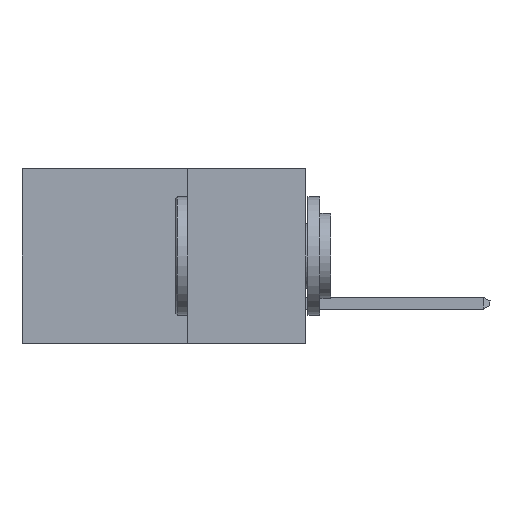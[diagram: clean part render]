
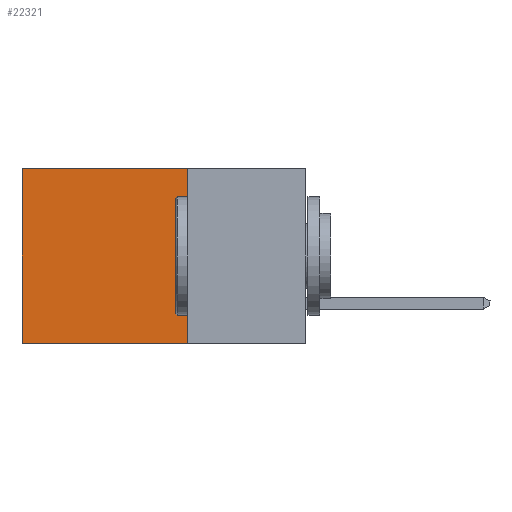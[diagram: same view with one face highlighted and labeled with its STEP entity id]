
A CAD part, left-side view. The second image highlights one B-rep face of the part: STEP entity #22321.
In plain terms, the highlighted planar face has unit normal (-1, 0, 0).
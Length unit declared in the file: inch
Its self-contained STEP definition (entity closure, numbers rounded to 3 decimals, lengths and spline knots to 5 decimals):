
#31 = AXIS2_PLACEMENT_3D ( 'NONE', #3484, #11914, #24074 ) ;
#255 = CARTESIAN_POINT ( 'NONE',  ( 0.298, 0.25, 0. ) ) ;
#766 = ORIENTED_EDGE ( 'NONE', *, *, #2165, .F. ) ;
#1873 = LINE ( 'NONE', #13272, #24845 ) ;
#2165 = EDGE_CURVE ( 'NONE', #18254, #13766, #9763, .T. ) ;
#2298 = ORIENTED_EDGE ( 'NONE', *, *, #14848, .F. ) ;
#3241 = DIRECTION ( 'NONE',  ( 0., 0., -1. ) ) ;
#3484 = CARTESIAN_POINT ( 'NONE',  ( 0.298, 0.25, 0. ) ) ;
#4947 = LINE ( 'NONE', #8418, #9716 ) ;
#5442 = EDGE_LOOP ( 'NONE', ( #11674, #766, #2298, #6397 ) ) ;
#6397 = ORIENTED_EDGE ( 'NONE', *, *, #21914, .T. ) ;
#8194 = EDGE_CURVE ( 'NONE', #22944, #13766, #1873, .T. ) ;
#8418 = CARTESIAN_POINT ( 'NONE',  ( 0.298, 0.25, 0. ) ) ;
#9106 = CARTESIAN_POINT ( 'NONE',  ( 0.298, 0.25, -0.37 ) ) ;
#9716 = VECTOR ( 'NONE', #18436, 39.37008 ) ;
#9763 = LINE ( 'NONE', #9106, #25762 ) ;
#10328 = CARTESIAN_POINT ( 'NONE',  ( 0.298, 0.6, -0.37 ) ) ;
#11137 = DIRECTION ( 'NONE',  ( 0., 1., 0. ) ) ;
#11674 = ORIENTED_EDGE ( 'NONE', *, *, #8194, .T. ) ;
#11914 = DIRECTION ( 'NONE',  ( 1., 0., 0. ) ) ;
#13272 = CARTESIAN_POINT ( 'NONE',  ( 0.298, 0.6, 0. ) ) ;
#13766 = VERTEX_POINT ( 'NONE', #10328 ) ;
#13927 = CARTESIAN_POINT ( 'NONE',  ( 0.298, 0.25, 0. ) ) ;
#14841 = FACE_OUTER_BOUND ( 'NONE', #5442, .T. ) ;
#14848 = EDGE_CURVE ( 'NONE', #23210, #18254, #24042, .T. ) ;
#15416 = VECTOR ( 'NONE', #20222, 39.37008 ) ;
#18254 = VERTEX_POINT ( 'NONE', #25111 ) ;
#18436 = DIRECTION ( 'NONE',  ( 0., 1., 0. ) ) ;
#19841 = PLANE ( 'NONE',  #31 ) ;
#20222 = DIRECTION ( 'NONE',  ( 0., 0., -1. ) ) ;
#21914 = EDGE_CURVE ( 'NONE', #23210, #22944, #4947, .T. ) ;
#22321 = ADVANCED_FACE ( 'NONE', ( #14841 ), #19841, .F. ) ;
#22944 = VERTEX_POINT ( 'NONE', #25562 ) ;
#23210 = VERTEX_POINT ( 'NONE', #13927 ) ;
#24042 = LINE ( 'NONE', #255, #15416 ) ;
#24074 = DIRECTION ( 'NONE',  ( 0., 0., -1. ) ) ;
#24845 = VECTOR ( 'NONE', #3241, 39.37008 ) ;
#25111 = CARTESIAN_POINT ( 'NONE',  ( 0.298, 0.25, -0.37 ) ) ;
#25562 = CARTESIAN_POINT ( 'NONE',  ( 0.298, 0.6, 0. ) ) ;
#25762 = VECTOR ( 'NONE', #11137, 39.37008 ) ;
